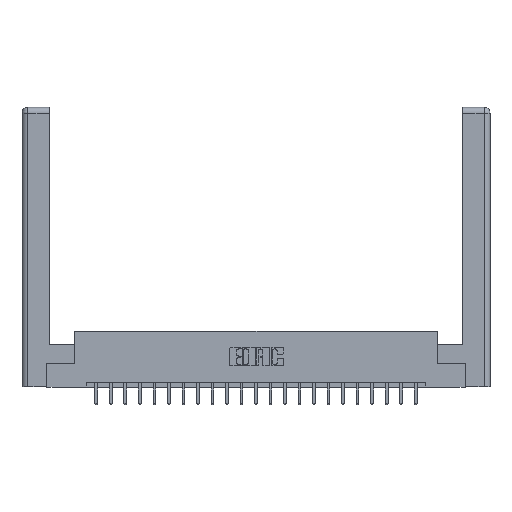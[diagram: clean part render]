
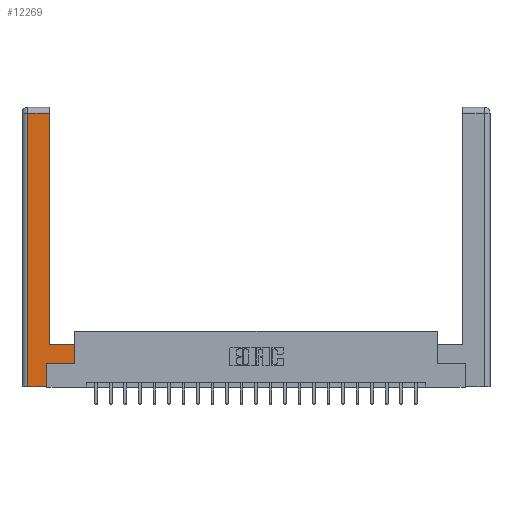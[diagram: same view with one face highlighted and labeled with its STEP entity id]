
A CAD part, top view. The second image highlights one B-rep face of the part: STEP entity #12269.
In plain terms, the highlighted planar face has unit normal (0, 0, 1).
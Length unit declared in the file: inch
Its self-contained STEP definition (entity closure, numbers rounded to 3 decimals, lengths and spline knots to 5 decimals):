
#246 = VECTOR ( 'NONE', #15433, 39.37008 ) ;
#784 = ORIENTED_EDGE ( 'NONE', *, *, #8166, .T. ) ;
#1187 = CARTESIAN_POINT ( 'NONE',  ( 0.265, 0.245, 0. ) ) ;
#1672 = LINE ( 'NONE', #11770, #14794 ) ;
#1827 = CARTESIAN_POINT ( 'NONE',  ( 0.295, 0.45, 0. ) ) ;
#3356 = VERTEX_POINT ( 'NONE', #20812 ) ;
#3514 = EDGE_CURVE ( 'NONE', #19943, #20220, #5624, .T. ) ;
#3765 = LINE ( 'NONE', #1187, #11883 ) ;
#4068 = ORIENTED_EDGE ( 'NONE', *, *, #20308, .T. ) ;
#4403 = EDGE_CURVE ( 'NONE', #6149, #19943, #1672, .T. ) ;
#4475 = VECTOR ( 'NONE', #7099, 39.37008 ) ;
#4748 = CARTESIAN_POINT ( 'NONE',  ( 0.565, 0.45, 0. ) ) ;
#4935 = ORIENTED_EDGE ( 'NONE', *, *, #4403, .T. ) ;
#4953 = CARTESIAN_POINT ( 'NONE',  ( 0.295, 0.45, 0. ) ) ;
#5116 = CARTESIAN_POINT ( 'NONE',  ( 0.565, 0.45, 0. ) ) ;
#5624 = LINE ( 'NONE', #5116, #12069 ) ;
#6087 = CARTESIAN_POINT ( 'NONE',  ( 0.0615, 0., 0. ) ) ;
#6149 = VERTEX_POINT ( 'NONE', #15441 ) ;
#6426 = DIRECTION ( 'NONE',  ( 1., 0., 0. ) ) ;
#7098 = ORIENTED_EDGE ( 'NONE', *, *, #21300, .T. ) ;
#7099 = DIRECTION ( 'NONE',  ( -1., 0., 0. ) ) ;
#7149 = DIRECTION ( 'NONE',  ( -1., 0., 0. ) ) ;
#8166 = EDGE_CURVE ( 'NONE', #3356, #6149, #3765, .T. ) ;
#8297 = LINE ( 'NONE', #19142, #246 ) ;
#8872 = LINE ( 'NONE', #9237, #13113 ) ;
#9237 = CARTESIAN_POINT ( 'NONE',  ( 0.0615, 0., 0. ) ) ;
#9561 = ORIENTED_EDGE ( 'NONE', *, *, #3514, .T. ) ;
#10058 = DIRECTION ( 'NONE',  ( 0., 1., 0. ) ) ;
#10534 = CARTESIAN_POINT ( 'NONE',  ( 0.295, 2.94, 0. ) ) ;
#10878 = LINE ( 'NONE', #17776, #4475 ) ;
#11279 = EDGE_CURVE ( 'NONE', #11829, #22052, #12279, .T. ) ;
#11659 = AXIS2_PLACEMENT_3D ( 'NONE', #21433, #19702, #7149 ) ;
#11770 = CARTESIAN_POINT ( 'NONE',  ( 0.565, 0.245, 0. ) ) ;
#11829 = VERTEX_POINT ( 'NONE', #1827 ) ;
#11883 = VECTOR ( 'NONE', #17067, 39.37008 ) ;
#12069 = VECTOR ( 'NONE', #15970, 39.37008 ) ;
#12269 = ADVANCED_FACE ( 'NONE', ( #13089 ), #21665, .F. ) ;
#12279 = LINE ( 'NONE', #17130, #21187 ) ;
#12497 = VECTOR ( 'NONE', #22819, 39.37008 ) ;
#12592 = ORIENTED_EDGE ( 'NONE', *, *, #11279, .T. ) ;
#12956 = DIRECTION ( 'NONE',  ( 0., -1., 0. ) ) ;
#13089 = FACE_OUTER_BOUND ( 'NONE', #17519, .T. ) ;
#13092 = LINE ( 'NONE', #4953, #12497 ) ;
#13113 = VECTOR ( 'NONE', #12956, 39.37008 ) ;
#14146 = VERTEX_POINT ( 'NONE', #6087 ) ;
#14794 = VECTOR ( 'NONE', #6426, 39.37008 ) ;
#15433 = DIRECTION ( 'NONE',  ( 1., 0., 0. ) ) ;
#15441 = CARTESIAN_POINT ( 'NONE',  ( 0.265, 0.245, 0. ) ) ;
#15970 = DIRECTION ( 'NONE',  ( 0., 1., 0. ) ) ;
#17067 = DIRECTION ( 'NONE',  ( 0., 1., 0. ) ) ;
#17130 = CARTESIAN_POINT ( 'NONE',  ( 0.295, 3., 0. ) ) ;
#17519 = EDGE_LOOP ( 'NONE', ( #12592, #17952, #4068, #18370, #784, #4935, #9561, #7098 ) ) ;
#17776 = CARTESIAN_POINT ( 'NONE',  ( 0.0615, 2.94, 0. ) ) ;
#17952 = ORIENTED_EDGE ( 'NONE', *, *, #19824, .T. ) ;
#18370 = ORIENTED_EDGE ( 'NONE', *, *, #21257, .T. ) ;
#19000 = CARTESIAN_POINT ( 'NONE',  ( 0.0615, 2.94, 0. ) ) ;
#19142 = CARTESIAN_POINT ( 'NONE',  ( 0.265, 0., 0. ) ) ;
#19702 = DIRECTION ( 'NONE',  ( 0., 0., -1. ) ) ;
#19824 = EDGE_CURVE ( 'NONE', #22052, #22692, #10878, .T. ) ;
#19943 = VERTEX_POINT ( 'NONE', #21456 ) ;
#20220 = VERTEX_POINT ( 'NONE', #4748 ) ;
#20308 = EDGE_CURVE ( 'NONE', #22692, #14146, #8872, .T. ) ;
#20812 = CARTESIAN_POINT ( 'NONE',  ( 0.265, 0., 0. ) ) ;
#21187 = VECTOR ( 'NONE', #10058, 39.37008 ) ;
#21257 = EDGE_CURVE ( 'NONE', #14146, #3356, #8297, .T. ) ;
#21300 = EDGE_CURVE ( 'NONE', #20220, #11829, #13092, .T. ) ;
#21433 = CARTESIAN_POINT ( 'NONE',  ( 0., 0., 0. ) ) ;
#21456 = CARTESIAN_POINT ( 'NONE',  ( 0.565, 0.245, 0. ) ) ;
#21665 = PLANE ( 'NONE',  #11659 ) ;
#22052 = VERTEX_POINT ( 'NONE', #10534 ) ;
#22692 = VERTEX_POINT ( 'NONE', #19000 ) ;
#22819 = DIRECTION ( 'NONE',  ( -1., 0., 0. ) ) ;
